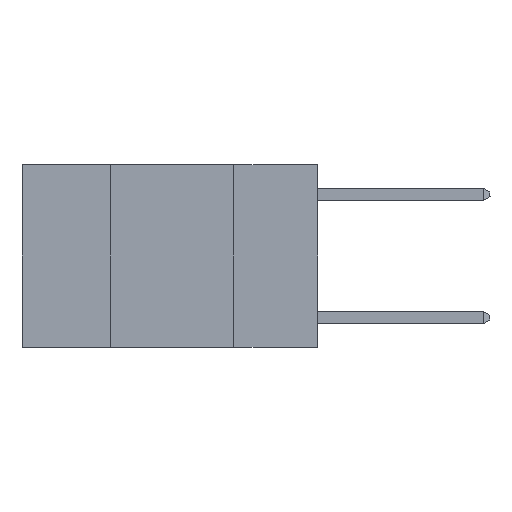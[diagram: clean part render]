
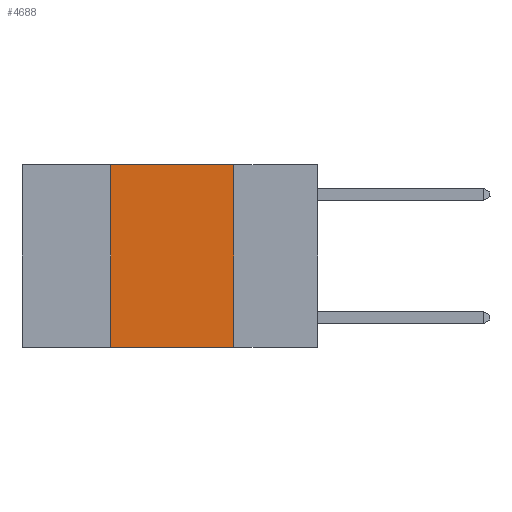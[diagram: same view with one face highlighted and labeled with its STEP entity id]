
A CAD part, left-side view. The second image highlights one B-rep face of the part: STEP entity #4688.
In plain terms, the highlighted planar face has unit normal (-1, 0, 0).
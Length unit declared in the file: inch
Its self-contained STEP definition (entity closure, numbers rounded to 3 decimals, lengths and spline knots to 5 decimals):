
#33 = LINE ( 'NONE', #8009, #8522 ) ;
#801 = AXIS2_PLACEMENT_3D ( 'NONE', #16807, #12825, #4854 ) ;
#1053 = DIRECTION ( 'NONE',  ( 0., 0., -1. ) ) ;
#1153 = ORIENTED_EDGE ( 'NONE', *, *, #4143, .F. ) ;
#1398 = ORIENTED_EDGE ( 'NONE', *, *, #13058, .T. ) ;
#2752 = CARTESIAN_POINT ( 'NONE',  ( 0., 0.17, -0.37 ) ) ;
#3050 = EDGE_CURVE ( 'NONE', #10003, #14980, #6634, .T. ) ;
#4143 = EDGE_CURVE ( 'NONE', #14539, #10003, #33, .T. ) ;
#4330 = PLANE ( 'NONE',  #801 ) ;
#4345 = CARTESIAN_POINT ( 'NONE',  ( 0., 0.6, 0. ) ) ;
#4688 = ADVANCED_FACE ( 'NONE', ( #5656 ), #4330, .F. ) ;
#4854 = DIRECTION ( 'NONE',  ( 0., 0., -1. ) ) ;
#4893 = VERTEX_POINT ( 'NONE', #2752 ) ;
#4973 = VECTOR ( 'NONE', #1053, 39.37008 ) ;
#5494 = EDGE_LOOP ( 'NONE', ( #6661, #12906, #1153, #1398 ) ) ;
#5530 = VECTOR ( 'NONE', #5967, 39.37008 ) ;
#5656 = FACE_OUTER_BOUND ( 'NONE', #5494, .T. ) ;
#5795 = CARTESIAN_POINT ( 'NONE',  ( 0., 0.6, -0.37 ) ) ;
#5967 = DIRECTION ( 'NONE',  ( 0., -1., 0. ) ) ;
#6634 = LINE ( 'NONE', #4345, #15090 ) ;
#6661 = ORIENTED_EDGE ( 'NONE', *, *, #13954, .F. ) ;
#7473 = CARTESIAN_POINT ( 'NONE',  ( 0., 0.42, 0. ) ) ;
#8009 = CARTESIAN_POINT ( 'NONE',  ( 0., 0.42, 0. ) ) ;
#8522 = VECTOR ( 'NONE', #13302, 39.37008 ) ;
#10003 = VERTEX_POINT ( 'NONE', #7473 ) ;
#12146 = DIRECTION ( 'NONE',  ( 0., -1., 0. ) ) ;
#12575 = LINE ( 'NONE', #15161, #4973 ) ;
#12825 = DIRECTION ( 'NONE',  ( 1., 0., 0. ) ) ;
#12906 = ORIENTED_EDGE ( 'NONE', *, *, #3050, .F. ) ;
#13058 = EDGE_CURVE ( 'NONE', #14539, #4893, #15230, .T. ) ;
#13242 = CARTESIAN_POINT ( 'NONE',  ( 0., 0.42, -0.37 ) ) ;
#13302 = DIRECTION ( 'NONE',  ( 0., 0., 1. ) ) ;
#13954 = EDGE_CURVE ( 'NONE', #14980, #4893, #12575, .T. ) ;
#14423 = CARTESIAN_POINT ( 'NONE',  ( 0., 0.17, 0. ) ) ;
#14539 = VERTEX_POINT ( 'NONE', #13242 ) ;
#14980 = VERTEX_POINT ( 'NONE', #14423 ) ;
#15090 = VECTOR ( 'NONE', #12146, 39.37008 ) ;
#15161 = CARTESIAN_POINT ( 'NONE',  ( 0., 0.17, 0. ) ) ;
#15230 = LINE ( 'NONE', #5795, #5530 ) ;
#16807 = CARTESIAN_POINT ( 'NONE',  ( 0., 0.6, 0. ) ) ;
